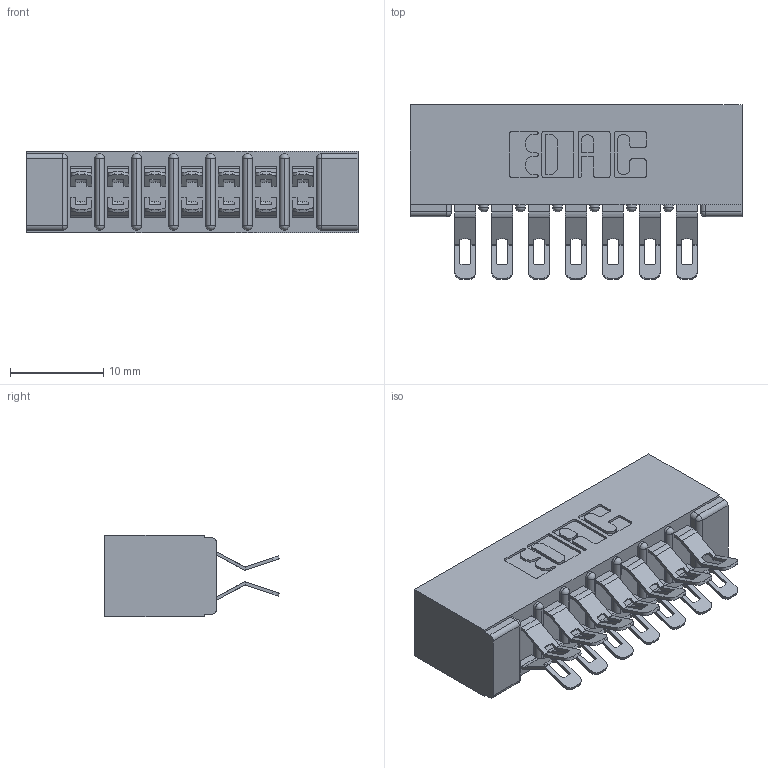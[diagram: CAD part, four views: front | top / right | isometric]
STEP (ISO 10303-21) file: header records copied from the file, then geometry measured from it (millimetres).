
FILE_DESCRIPTION (( 'STEP AP203' ), '1' );
FILE_NAME ('307-014-455-201.STEP', '2020-09-28T16:04:30', ( '' ), ( '' ), 'SwSTEP 2.0', 'SolidWorks 2020', '' );
FILE_SCHEMA (( 'CONFIG_CONTROL_DESIGN' ));
Length unit declared in the file: inch
Products named in the file (3): 307-290-001_555; 307 Part_No Mounting Lugs; 307-014-455-201
Assembly tree (15 placements, depth 2):
  307-014-455-201
    307 Part_No Mounting Lugs
    307-290-001_555  x14
Bounding box: 35.61 x 18.75 x 8.71 mm (x, y, z)
Volume: 2605.8 mm3; surface area: 4521.4 mm2
Topology: 15 solids, 15 shells, 972 faces, 2833 edges, 1846 vertices
Faces by surface type: plane 542, cylinder 414, sphere 16
Entity records: 10799 total; most frequent: CARTESIAN_POINT 1779, DIRECTION 1764, ORIENTED_EDGE 1760, EDGE_CURVE 880, LINE 650, VECTOR 650, VERTEX_POINT 572, AXIS2_PLACEMENT_3D 557
